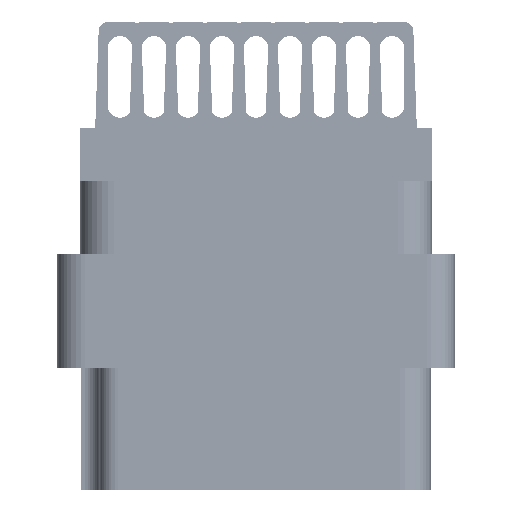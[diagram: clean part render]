
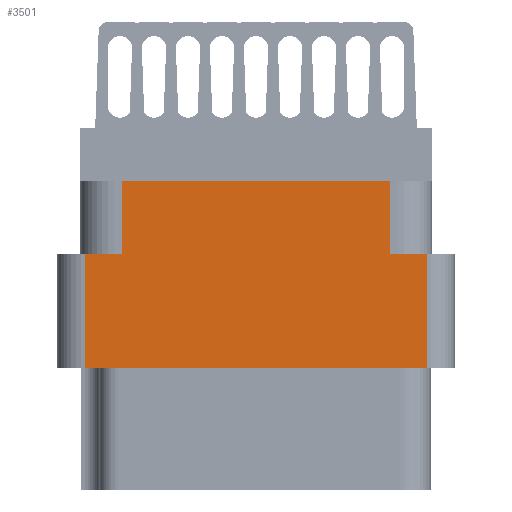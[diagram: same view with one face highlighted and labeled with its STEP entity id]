
A CAD part, left-side view. The second image highlights one B-rep face of the part: STEP entity #3501.
In plain terms, the highlighted planar face has unit normal (-1, 0, 0).
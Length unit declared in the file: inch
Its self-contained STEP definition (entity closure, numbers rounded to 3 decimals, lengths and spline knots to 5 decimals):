
#1495 = DIRECTION ( 'NONE',  ( 0., 0., 1. ) ) ;
#2320 = LINE ( 'NONE', #31273, #17813 ) ;
#2374 = EDGE_CURVE ( 'NONE', #43484, #21000, #10317, .T. ) ;
#2834 = ORIENTED_EDGE ( 'NONE', *, *, #20935, .F. ) ;
#3216 = CARTESIAN_POINT ( 'NONE',  ( -1.296, 0.376, -0.798 ) ) ;
#3445 = LINE ( 'NONE', #49145, #48105 ) ;
#3501 = ADVANCED_FACE ( 'NONE', ( #50505 ), #15890, .T. ) ;
#3847 = CARTESIAN_POINT ( 'NONE',  ( -1.296, 0.376, -0.277 ) ) ;
#4061 = LINE ( 'NONE', #19467, #42478 ) ;
#4247 = CARTESIAN_POINT ( 'NONE',  ( -1.296, 0.438, -0.117 ) ) ;
#5698 = EDGE_CURVE ( 'NONE', #40520, #21000, #3445, .T. ) ;
#5934 = EDGE_CURVE ( 'NONE', #43854, #31513, #4061, .T. ) ;
#6807 = CARTESIAN_POINT ( 'NONE',  ( -1.296, -0.296, -0.277 ) ) ;
#8614 = VERTEX_POINT ( 'NONE', #12385 ) ;
#9800 = ORIENTED_EDGE ( 'NONE', *, *, #45546, .F. ) ;
#10317 = LINE ( 'NONE', #4247, #47568 ) ;
#10418 = ORIENTED_EDGE ( 'NONE', *, *, #5934, .T. ) ;
#11839 = DIRECTION ( 'NONE',  ( 0., 0., 1. ) ) ;
#11852 = CARTESIAN_POINT ( 'NONE',  ( -1.296, -0.376, -0.529 ) ) ;
#12385 = CARTESIAN_POINT ( 'NONE',  ( -1.296, 0.296, -0.277 ) ) ;
#13033 = CARTESIAN_POINT ( 'NONE',  ( -1.296, 0., -0.529 ) ) ;
#13463 = VECTOR ( 'NONE', #26175, 39.37008 ) ;
#13504 = CARTESIAN_POINT ( 'NONE',  ( -1.296, -0.296, -0.117 ) ) ;
#15039 = VECTOR ( 'NONE', #44936, 39.37008 ) ;
#15692 = DIRECTION ( 'NONE',  ( 0., 0., -1. ) ) ;
#15890 = PLANE ( 'NONE',  #25509 ) ;
#16335 = DIRECTION ( 'NONE',  ( 0., -1., 0. ) ) ;
#17759 = CARTESIAN_POINT ( 'NONE',  ( -1.296, 0.296, -0.117 ) ) ;
#17813 = VECTOR ( 'NONE', #11839, 39.37008 ) ;
#18312 = ORIENTED_EDGE ( 'NONE', *, *, #5698, .T. ) ;
#18757 = CARTESIAN_POINT ( 'NONE',  ( -1.296, 0., -0.277 ) ) ;
#19467 = CARTESIAN_POINT ( 'NONE',  ( -1.296, -0.376, -0.798 ) ) ;
#20622 = CARTESIAN_POINT ( 'NONE',  ( -1.296, 0., -0.277 ) ) ;
#20935 = EDGE_CURVE ( 'NONE', #40520, #31513, #30796, .T. ) ;
#21000 = VERTEX_POINT ( 'NONE', #13504 ) ;
#22205 = CARTESIAN_POINT ( 'NONE',  ( -1.296, 0.376, -0.529 ) ) ;
#23600 = ORIENTED_EDGE ( 'NONE', *, *, #29189, .F. ) ;
#25271 = ORIENTED_EDGE ( 'NONE', *, *, #48705, .F. ) ;
#25509 = AXIS2_PLACEMENT_3D ( 'NONE', #43977, #31831, #47944 ) ;
#26175 = DIRECTION ( 'NONE',  ( 0., -1., 0. ) ) ;
#28226 = ORIENTED_EDGE ( 'NONE', *, *, #50169, .T. ) ;
#28376 = LINE ( 'NONE', #18757, #13463 ) ;
#29189 = EDGE_CURVE ( 'NONE', #42760, #8614, #28376, .T. ) ;
#30796 = LINE ( 'NONE', #20622, #32641 ) ;
#31273 = CARTESIAN_POINT ( 'NONE',  ( -1.296, 0.296, -0.277 ) ) ;
#31513 = VERTEX_POINT ( 'NONE', #34706 ) ;
#31831 = DIRECTION ( 'NONE',  ( -1., 0., 0. ) ) ;
#32122 = DIRECTION ( 'NONE',  ( 0., -1., 0. ) ) ;
#32374 = VERTEX_POINT ( 'NONE', #22205 ) ;
#32641 = VECTOR ( 'NONE', #16335, 39.37008 ) ;
#34706 = CARTESIAN_POINT ( 'NONE',  ( -1.296, -0.376, -0.277 ) ) ;
#37181 = EDGE_LOOP ( 'NONE', ( #23600, #28226, #25271, #10418, #2834, #18312, #47623, #9800 ) ) ;
#40520 = VERTEX_POINT ( 'NONE', #6807 ) ;
#41494 = LINE ( 'NONE', #3216, #50803 ) ;
#42478 = VECTOR ( 'NONE', #47239, 39.37008 ) ;
#42760 = VERTEX_POINT ( 'NONE', #3847 ) ;
#43484 = VERTEX_POINT ( 'NONE', #17759 ) ;
#43854 = VERTEX_POINT ( 'NONE', #11852 ) ;
#43977 = CARTESIAN_POINT ( 'NONE',  ( -1.296, -0.438, -0.798 ) ) ;
#44936 = DIRECTION ( 'NONE',  ( 0., 1., 0. ) ) ;
#45431 = LINE ( 'NONE', #13033, #15039 ) ;
#45546 = EDGE_CURVE ( 'NONE', #8614, #43484, #2320, .T. ) ;
#47239 = DIRECTION ( 'NONE',  ( 0., 0., 1. ) ) ;
#47568 = VECTOR ( 'NONE', #32122, 39.37008 ) ;
#47623 = ORIENTED_EDGE ( 'NONE', *, *, #2374, .F. ) ;
#47944 = DIRECTION ( 'NONE',  ( 0., 0., 1. ) ) ;
#48105 = VECTOR ( 'NONE', #1495, 39.37008 ) ;
#48705 = EDGE_CURVE ( 'NONE', #43854, #32374, #45431, .T. ) ;
#49145 = CARTESIAN_POINT ( 'NONE',  ( -1.296, -0.296, -0.277 ) ) ;
#50169 = EDGE_CURVE ( 'NONE', #42760, #32374, #41494, .T. ) ;
#50505 = FACE_OUTER_BOUND ( 'NONE', #37181, .T. ) ;
#50803 = VECTOR ( 'NONE', #15692, 39.37008 ) ;
